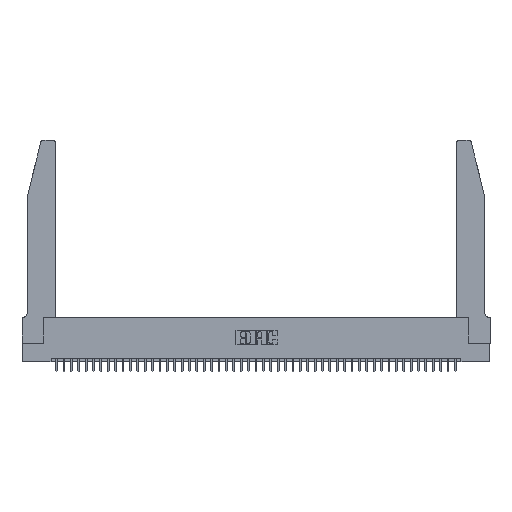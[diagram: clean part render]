
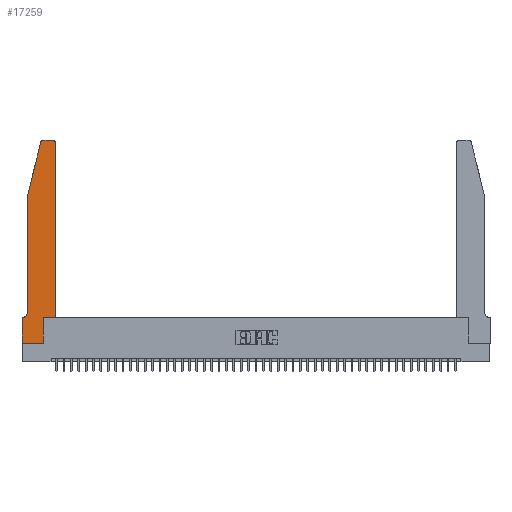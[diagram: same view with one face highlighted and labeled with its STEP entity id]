
A CAD part, top view. The second image highlights one B-rep face of the part: STEP entity #17259.
In plain terms, the highlighted planar face has unit normal (0, 0, 1).
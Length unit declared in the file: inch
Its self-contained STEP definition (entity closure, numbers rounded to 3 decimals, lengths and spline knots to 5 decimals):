
#176 = DIRECTION ( 'NONE',  ( 0., -1., 0. ) ) ;
#1761 = DIRECTION ( 'NONE',  ( 0., 0., 1. ) ) ;
#1833 = VERTEX_POINT ( 'NONE', #16343 ) ;
#2353 = DIRECTION ( 'NONE',  ( 0., 0., 1. ) ) ;
#3467 = EDGE_CURVE ( 'NONE', #23651, #43823, #30519, .T. ) ;
#3953 = DIRECTION ( 'NONE',  ( 1., 0., 0. ) ) ;
#4105 = ORIENTED_EDGE ( 'NONE', *, *, #7132, .T. ) ;
#4546 = LINE ( 'NONE', #43082, #22450 ) ;
#5066 = ORIENTED_EDGE ( 'NONE', *, *, #3467, .T. ) ;
#5816 = CARTESIAN_POINT ( 'NONE',  ( 0.0055, 0.42, 0.37 ) ) ;
#6092 = LINE ( 'NONE', #7453, #45083 ) ;
#6247 = EDGE_CURVE ( 'NONE', #13567, #14206, #6092, .T. ) ;
#7132 = EDGE_CURVE ( 'NONE', #43823, #1833, #18879, .T. ) ;
#7453 = CARTESIAN_POINT ( 'NONE',  ( 0.4505, 0.35, 0.37 ) ) ;
#7813 = ORIENTED_EDGE ( 'NONE', *, *, #38439, .T. ) ;
#8980 = ORIENTED_EDGE ( 'NONE', *, *, #36957, .T. ) ;
#9150 = VECTOR ( 'NONE', #34761, 39.37008 ) ;
#9404 = DIRECTION ( 'NONE',  ( -1., 0., 0. ) ) ;
#9772 = CARTESIAN_POINT ( 'NONE',  ( 0.4505, 2.72, 0.37 ) ) ;
#10067 = EDGE_CURVE ( 'NONE', #26976, #11705, #10258, .T. ) ;
#10258 = LINE ( 'NONE', #31228, #9150 ) ;
#10756 = VECTOR ( 'NONE', #45000, 39.37008 ) ;
#11087 = VERTEX_POINT ( 'NONE', #33301 ) ;
#11473 = VERTEX_POINT ( 'NONE', #15997 ) ;
#11588 = EDGE_LOOP ( 'NONE', ( #27660, #22688, #32218, #5066, #4105, #13608, #26116, #19487, #19305, #8980, #45805, #7813 ) ) ;
#11614 = EDGE_CURVE ( 'NONE', #35246, #23651, #42431, .T. ) ;
#11705 = VERTEX_POINT ( 'NONE', #35124 ) ;
#11916 = LINE ( 'NONE', #41448, #10756 ) ;
#13312 = DIRECTION ( 'NONE',  ( -0.239, -0.971, 0. ) ) ;
#13567 = VERTEX_POINT ( 'NONE', #42216 ) ;
#13608 = ORIENTED_EDGE ( 'NONE', *, *, #16110, .T. ) ;
#14206 = VERTEX_POINT ( 'NONE', #9772 ) ;
#14502 = CARTESIAN_POINT ( 'NONE',  ( 0.0755, 2., 0.37 ) ) ;
#15841 = CARTESIAN_POINT ( 'NONE',  ( 0.0755, 2., 0.37 ) ) ;
#15997 = CARTESIAN_POINT ( 'NONE',  ( 0., 0., 0.37 ) ) ;
#16110 = EDGE_CURVE ( 'NONE', #1833, #33389, #41053, .T. ) ;
#16343 = CARTESIAN_POINT ( 'NONE',  ( 0.0055, 0.35, 0.37 ) ) ;
#16574 = CARTESIAN_POINT ( 'NONE',  ( 0.0755, 0.42, 0.37 ) ) ;
#17125 = CARTESIAN_POINT ( 'NONE',  ( 0., 0.35, 0.37 ) ) ;
#17129 = CARTESIAN_POINT ( 'NONE',  ( 0.25487, 2.72718, 0.37 ) ) ;
#17169 = EDGE_CURVE ( 'NONE', #33389, #11473, #25942, .T. ) ;
#17259 = ADVANCED_FACE ( 'NONE', ( #21447 ), #36463, .T. ) ;
#18449 = EDGE_CURVE ( 'NONE', #11087, #35246, #43036, .T. ) ;
#18682 = DIRECTION ( 'NONE',  ( 0., 0., 1. ) ) ;
#18879 = CIRCLE ( 'NONE', #28811, 0.07 ) ;
#18945 = CARTESIAN_POINT ( 'NONE',  ( 0.0755, 0.35, 0.37 ) ) ;
#19305 = ORIENTED_EDGE ( 'NONE', *, *, #10067, .T. ) ;
#19487 = ORIENTED_EDGE ( 'NONE', *, *, #30511, .T. ) ;
#20982 = VECTOR ( 'NONE', #176, 39.37008 ) ;
#21447 = FACE_OUTER_BOUND ( 'NONE', #11588, .T. ) ;
#21646 = CARTESIAN_POINT ( 'NONE',  ( 0., 0., 0.37 ) ) ;
#22450 = VECTOR ( 'NONE', #3953, 39.37008 ) ;
#22688 = ORIENTED_EDGE ( 'NONE', *, *, #18449, .T. ) ;
#23218 = CARTESIAN_POINT ( 'NONE',  ( 0.4205, 2.72, 0.37 ) ) ;
#23651 = VERTEX_POINT ( 'NONE', #15841 ) ;
#23810 = CARTESIAN_POINT ( 'NONE',  ( 0.284, 2.72, 0.37 ) ) ;
#23900 = CARTESIAN_POINT ( 'NONE',  ( 0.0755, 2., 0.37 ) ) ;
#25229 = DIRECTION ( 'NONE',  ( 0., -1., 0. ) ) ;
#25942 = LINE ( 'NONE', #21646, #43683 ) ;
#26116 = ORIENTED_EDGE ( 'NONE', *, *, #17169, .T. ) ;
#26976 = VERTEX_POINT ( 'NONE', #41633 ) ;
#27394 = VECTOR ( 'NONE', #30505, 39.37008 ) ;
#27423 = DIRECTION ( 'NONE',  ( 1., 0., 0. ) ) ;
#27660 = ORIENTED_EDGE ( 'NONE', *, *, #32348, .T. ) ;
#28456 = CARTESIAN_POINT ( 'NONE',  ( 0.4205, 2.75, 0.37 ) ) ;
#28524 = LINE ( 'NONE', #41168, #27394 ) ;
#28811 = AXIS2_PLACEMENT_3D ( 'NONE', #5816, #30858, #9404 ) ;
#30505 = DIRECTION ( 'NONE',  ( -1., 0., 0. ) ) ;
#30511 = EDGE_CURVE ( 'NONE', #11473, #26976, #11916, .T. ) ;
#30519 = LINE ( 'NONE', #14502, #20982 ) ;
#30858 = DIRECTION ( 'NONE',  ( 0., 0., -1. ) ) ;
#31228 = CARTESIAN_POINT ( 'NONE',  ( 0.2865, 0.35, 0.37 ) ) ;
#31641 = VECTOR ( 'NONE', #40271, 39.37008 ) ;
#32218 = ORIENTED_EDGE ( 'NONE', *, *, #11614, .T. ) ;
#32348 = EDGE_CURVE ( 'NONE', #39947, #11087, #28524, .T. ) ;
#32350 = AXIS2_PLACEMENT_3D ( 'NONE', #40012, #18682, #43534 ) ;
#32918 = AXIS2_PLACEMENT_3D ( 'NONE', #23218, #1761, #36134 ) ;
#33044 = VECTOR ( 'NONE', #13312, 39.37008 ) ;
#33301 = CARTESIAN_POINT ( 'NONE',  ( 0.284, 2.75, 0.37 ) ) ;
#33389 = VERTEX_POINT ( 'NONE', #17125 ) ;
#34761 = DIRECTION ( 'NONE',  ( 0., 1., 0. ) ) ;
#35124 = CARTESIAN_POINT ( 'NONE',  ( 0.2865, 0.35, 0.37 ) ) ;
#35246 = VERTEX_POINT ( 'NONE', #17129 ) ;
#35871 = DIRECTION ( 'NONE',  ( 0., 1., 0. ) ) ;
#36134 = DIRECTION ( 'NONE',  ( 1., 0., 0. ) ) ;
#36463 = PLANE ( 'NONE',  #32350 ) ;
#36957 = EDGE_CURVE ( 'NONE', #11705, #13567, #4546, .T. ) ;
#38439 = EDGE_CURVE ( 'NONE', #14206, #39947, #45736, .T. ) ;
#39947 = VERTEX_POINT ( 'NONE', #28456 ) ;
#40012 = CARTESIAN_POINT ( 'NONE',  ( 0., 0.35, 0.37 ) ) ;
#40271 = DIRECTION ( 'NONE',  ( -1., 0., 0. ) ) ;
#41053 = LINE ( 'NONE', #18945, #31641 ) ;
#41168 = CARTESIAN_POINT ( 'NONE',  ( 0.2605, 2.75, 0.37 ) ) ;
#41448 = CARTESIAN_POINT ( 'NONE',  ( 0., 0., 0.37 ) ) ;
#41548 = AXIS2_PLACEMENT_3D ( 'NONE', #23810, #2353, #27423 ) ;
#41633 = CARTESIAN_POINT ( 'NONE',  ( 0.2865, 0., 0.37 ) ) ;
#42216 = CARTESIAN_POINT ( 'NONE',  ( 0.4505, 0.35, 0.37 ) ) ;
#42431 = LINE ( 'NONE', #23900, #33044 ) ;
#43036 = CIRCLE ( 'NONE', #41548, 0.03 ) ;
#43082 = CARTESIAN_POINT ( 'NONE',  ( 0.4505, 0.35, 0.37 ) ) ;
#43534 = DIRECTION ( 'NONE',  ( 1., 0., 0. ) ) ;
#43683 = VECTOR ( 'NONE', #25229, 39.37008 ) ;
#43823 = VERTEX_POINT ( 'NONE', #16574 ) ;
#45000 = DIRECTION ( 'NONE',  ( 1., 0., 0. ) ) ;
#45083 = VECTOR ( 'NONE', #35871, 39.37008 ) ;
#45736 = CIRCLE ( 'NONE', #32918, 0.03 ) ;
#45805 = ORIENTED_EDGE ( 'NONE', *, *, #6247, .T. ) ;
